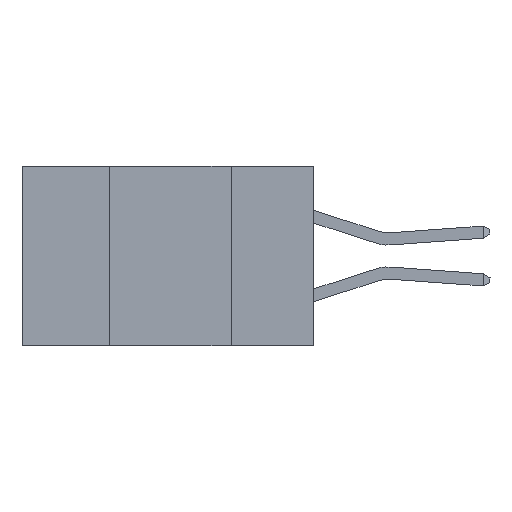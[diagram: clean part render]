
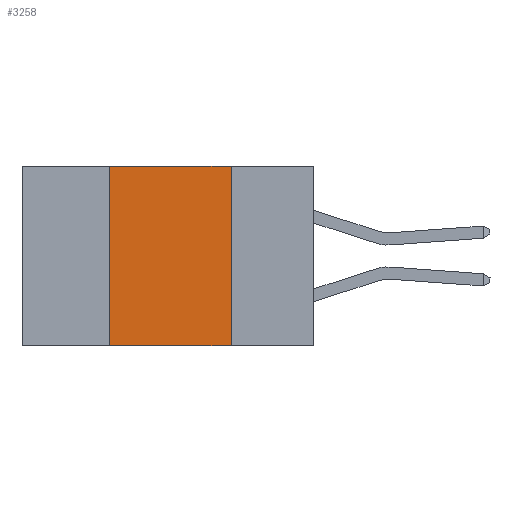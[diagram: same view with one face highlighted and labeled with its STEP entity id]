
A CAD part, left-side view. The second image highlights one B-rep face of the part: STEP entity #3258.
In plain terms, the highlighted planar face has unit normal (-1, 0, 0).
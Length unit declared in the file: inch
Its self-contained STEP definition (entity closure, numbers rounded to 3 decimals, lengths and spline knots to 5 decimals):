
#132 = CARTESIAN_POINT ( 'NONE',  ( 0., 0.17, 0. ) ) ;
#310 = CARTESIAN_POINT ( 'NONE',  ( 0., 0.6, -0.37 ) ) ;
#526 = CARTESIAN_POINT ( 'NONE',  ( 0., 0.6, 0. ) ) ;
#1719 = EDGE_CURVE ( 'NONE', #9931, #14878, #7792, .T. ) ;
#1793 = VERTEX_POINT ( 'NONE', #132 ) ;
#1813 = DIRECTION ( 'NONE',  ( 0., 0., -1. ) ) ;
#2061 = EDGE_LOOP ( 'NONE', ( #8524, #13378, #10052, #4671 ) ) ;
#2567 = AXIS2_PLACEMENT_3D ( 'NONE', #5557, #14437, #14616 ) ;
#3258 = ADVANCED_FACE ( 'NONE', ( #15745 ), #15293, .F. ) ;
#3610 = CARTESIAN_POINT ( 'NONE',  ( 0., 0.42, 0. ) ) ;
#4620 = CARTESIAN_POINT ( 'NONE',  ( 0., 0.17, -0.37 ) ) ;
#4671 = ORIENTED_EDGE ( 'NONE', *, *, #1719, .T. ) ;
#5291 = CARTESIAN_POINT ( 'NONE',  ( 0., 0.42, 0. ) ) ;
#5557 = CARTESIAN_POINT ( 'NONE',  ( 0., 0.6, 0. ) ) ;
#5889 = LINE ( 'NONE', #526, #7874 ) ;
#6982 = CARTESIAN_POINT ( 'NONE',  ( 0., 0.17, 0. ) ) ;
#7792 = LINE ( 'NONE', #310, #9212 ) ;
#7874 = VECTOR ( 'NONE', #8453, 39.37008 ) ;
#8453 = DIRECTION ( 'NONE',  ( 0., -1., 0. ) ) ;
#8524 = ORIENTED_EDGE ( 'NONE', *, *, #11631, .F. ) ;
#9212 = VECTOR ( 'NONE', #10660, 39.37008 ) ;
#9931 = VERTEX_POINT ( 'NONE', #11759 ) ;
#10052 = ORIENTED_EDGE ( 'NONE', *, *, #13311, .F. ) ;
#10660 = DIRECTION ( 'NONE',  ( 0., -1., 0. ) ) ;
#10790 = LINE ( 'NONE', #6982, #12444 ) ;
#11631 = EDGE_CURVE ( 'NONE', #1793, #14878, #10790, .T. ) ;
#11759 = CARTESIAN_POINT ( 'NONE',  ( 0., 0.42, -0.37 ) ) ;
#12444 = VECTOR ( 'NONE', #1813, 39.37008 ) ;
#12996 = LINE ( 'NONE', #5291, #16619 ) ;
#13019 = DIRECTION ( 'NONE',  ( 0., 0., 1. ) ) ;
#13311 = EDGE_CURVE ( 'NONE', #9931, #15590, #12996, .T. ) ;
#13378 = ORIENTED_EDGE ( 'NONE', *, *, #15935, .F. ) ;
#14437 = DIRECTION ( 'NONE',  ( 1., 0., 0. ) ) ;
#14616 = DIRECTION ( 'NONE',  ( 0., 0., -1. ) ) ;
#14878 = VERTEX_POINT ( 'NONE', #4620 ) ;
#15293 = PLANE ( 'NONE',  #2567 ) ;
#15590 = VERTEX_POINT ( 'NONE', #3610 ) ;
#15745 = FACE_OUTER_BOUND ( 'NONE', #2061, .T. ) ;
#15935 = EDGE_CURVE ( 'NONE', #15590, #1793, #5889, .T. ) ;
#16619 = VECTOR ( 'NONE', #13019, 39.37008 ) ;
